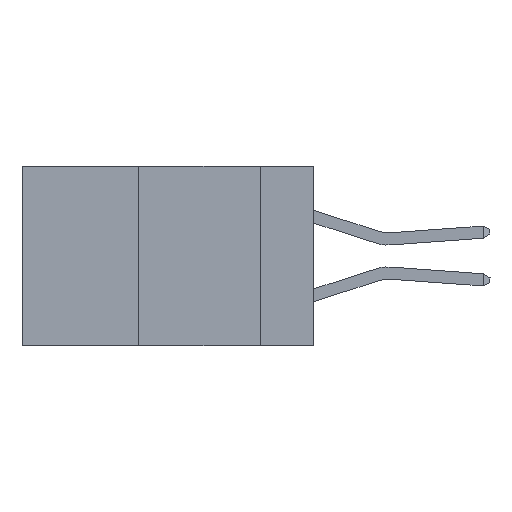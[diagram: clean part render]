
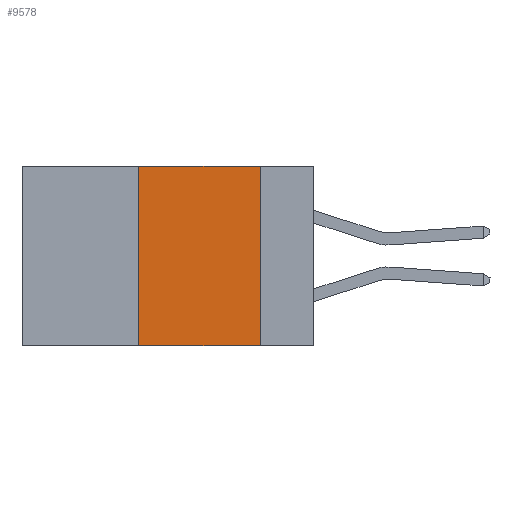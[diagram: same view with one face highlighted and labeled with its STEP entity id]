
A CAD part, left-side view. The second image highlights one B-rep face of the part: STEP entity #9578.
In plain terms, the highlighted planar face has unit normal (-1, 0, 0).
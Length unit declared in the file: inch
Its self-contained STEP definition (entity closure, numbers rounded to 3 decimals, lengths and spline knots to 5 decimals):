
#1001 = DIRECTION ( 'NONE',  ( 0., -1., 0. ) ) ;
#1391 = DIRECTION ( 'NONE',  ( 0., -1., 0. ) ) ;
#4171 = DIRECTION ( 'NONE',  ( 1., 0., 0. ) ) ;
#6100 = EDGE_CURVE ( 'NONE', #15309, #30056, #32564, .T. ) ;
#6306 = VERTEX_POINT ( 'NONE', #37836 ) ;
#7125 = EDGE_LOOP ( 'NONE', ( #14495, #12302, #22576, #20637 ) ) ;
#7367 = VECTOR ( 'NONE', #1001, 39.37008 ) ;
#9578 = ADVANCED_FACE ( 'NONE', ( #31767 ), #16774, .F. ) ;
#10563 = EDGE_CURVE ( 'NONE', #15309, #35379, #16826, .T. ) ;
#12302 = ORIENTED_EDGE ( 'NONE', *, *, #13224, .F. ) ;
#13224 = EDGE_CURVE ( 'NONE', #30056, #6306, #25776, .T. ) ;
#13781 = CARTESIAN_POINT ( 'NONE',  ( 0., 0.36, 0. ) ) ;
#14490 = DIRECTION ( 'NONE',  ( 0., 0., 1. ) ) ;
#14495 = ORIENTED_EDGE ( 'NONE', *, *, #30701, .F. ) ;
#15309 = VERTEX_POINT ( 'NONE', #27406 ) ;
#16774 = PLANE ( 'NONE',  #27072 ) ;
#16826 = LINE ( 'NONE', #18145, #17857 ) ;
#17857 = VECTOR ( 'NONE', #1391, 39.37008 ) ;
#18145 = CARTESIAN_POINT ( 'NONE',  ( 0., 0.6, -0.37 ) ) ;
#20637 = ORIENTED_EDGE ( 'NONE', *, *, #10563, .T. ) ;
#21560 = VECTOR ( 'NONE', #35734, 39.37008 ) ;
#22576 = ORIENTED_EDGE ( 'NONE', *, *, #6100, .F. ) ;
#22590 = LINE ( 'NONE', #40102, #21560 ) ;
#24919 = CARTESIAN_POINT ( 'NONE',  ( 0., 0.36, 0. ) ) ;
#24928 = VECTOR ( 'NONE', #14490, 39.37008 ) ;
#25776 = LINE ( 'NONE', #30480, #7367 ) ;
#27072 = AXIS2_PLACEMENT_3D ( 'NONE', #33309, #4171, #39847 ) ;
#27406 = CARTESIAN_POINT ( 'NONE',  ( 0., 0.36, -0.37 ) ) ;
#28646 = CARTESIAN_POINT ( 'NONE',  ( 0., 0.11, -0.37 ) ) ;
#30056 = VERTEX_POINT ( 'NONE', #24919 ) ;
#30480 = CARTESIAN_POINT ( 'NONE',  ( 0., 0.6, 0. ) ) ;
#30701 = EDGE_CURVE ( 'NONE', #6306, #35379, #22590, .T. ) ;
#31767 = FACE_OUTER_BOUND ( 'NONE', #7125, .T. ) ;
#32564 = LINE ( 'NONE', #13781, #24928 ) ;
#33309 = CARTESIAN_POINT ( 'NONE',  ( 0., 0.6, 0. ) ) ;
#35379 = VERTEX_POINT ( 'NONE', #28646 ) ;
#35734 = DIRECTION ( 'NONE',  ( 0., 0., -1. ) ) ;
#37836 = CARTESIAN_POINT ( 'NONE',  ( 0., 0.11, 0. ) ) ;
#39847 = DIRECTION ( 'NONE',  ( 0., 0., -1. ) ) ;
#40102 = CARTESIAN_POINT ( 'NONE',  ( 0., 0.11, 0. ) ) ;
